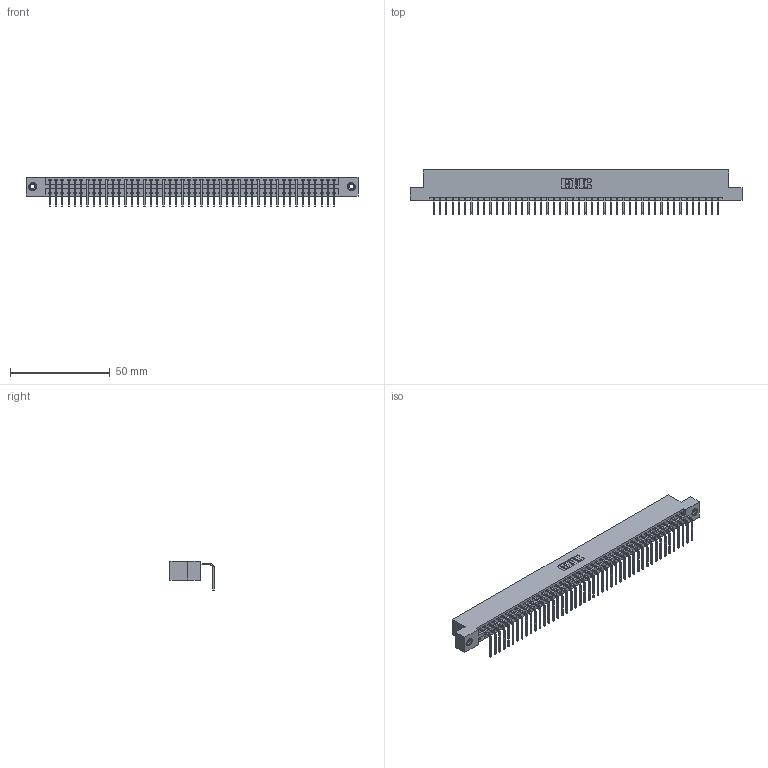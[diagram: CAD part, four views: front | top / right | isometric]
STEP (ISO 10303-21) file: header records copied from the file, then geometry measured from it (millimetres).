
FILE_DESCRIPTION (( 'STEP AP203' ), '1' );
FILE_NAME ('346-046-558-108.STEP', '2018-08-25T06:28:33', ( '' ), ( '' ), 'SwSTEP 2.0', 'SolidWorks 2016', '' );
FILE_SCHEMA (( 'CONFIG_CONTROL_DESIGN' ));
Length unit declared in the file: inch
Products named in the file (4): 346 Part_Flush Mounting Lugs - 0.156 Dia-TI; 345-292-001_558 Tail - 2; 345-250-001_345-250-003-102; 346-046-558-108
Assembly tree (49 placements, depth 2):
  346-046-558-108
    346 Part_Flush Mounting Lugs - 0.156 Dia-TI
    345-292-001_558 Tail - 2  x46
    345-250-001_345-250-003-102  x2
Bounding box: 166.62 x 22.16 x 14.73 mm (x, y, z)
Volume: 16123.9 mm3; surface area: 21132.1 mm2
Topology: 49 solids, 49 shells, 2942 faces, 8837 edges, 5822 vertices
Faces by surface type: plane 2040, cylinder 886, cone 12, torus 4
Entity records: 29280 total; most frequent: CARTESIAN_POINT 5001, ORIENTED_EDGE 4974, DIRECTION 4433, EDGE_CURVE 2487, LINE 2151, VECTOR 2151, VERTEX_POINT 1652, AXIS2_PLACEMENT_3D 1141
